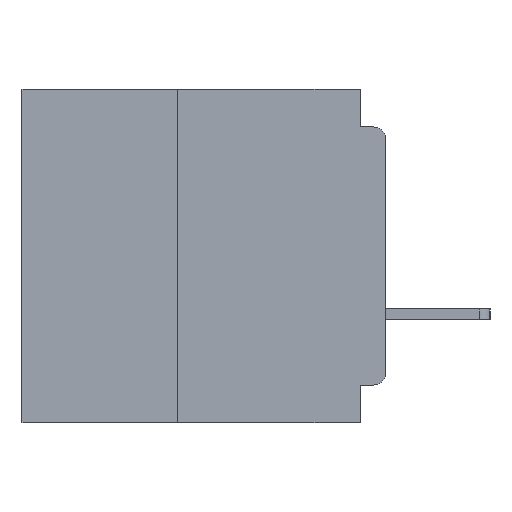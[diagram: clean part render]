
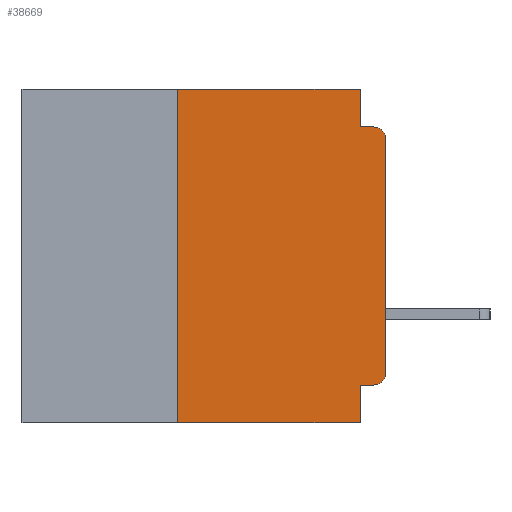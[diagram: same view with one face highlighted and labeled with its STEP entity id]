
A CAD part, left-side view. The second image highlights one B-rep face of the part: STEP entity #38669.
In plain terms, the highlighted planar face has unit normal (-1, 0, 0).
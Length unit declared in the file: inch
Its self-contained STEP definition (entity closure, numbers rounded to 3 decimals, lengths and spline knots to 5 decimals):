
#1066 = CARTESIAN_POINT ( 'NONE',  ( 0., 0., -0.34 ) ) ;
#1947 = CARTESIAN_POINT ( 'NONE',  ( 0., 0.015, -0.355 ) ) ;
#2549 = DIRECTION ( 'NONE',  ( 0., 1., 0. ) ) ;
#3871 = EDGE_CURVE ( 'NONE', #40493, #19593, #13077, .T. ) ;
#4019 = CARTESIAN_POINT ( 'NONE',  ( 0., 0.437, 0. ) ) ;
#4484 = LINE ( 'NONE', #27538, #34651 ) ;
#5518 = CARTESIAN_POINT ( 'NONE',  ( 0., 0.031, -0.045 ) ) ;
#5883 = ORIENTED_EDGE ( 'NONE', *, *, #23034, .T. ) ;
#6150 = VERTEX_POINT ( 'NONE', #48882 ) ;
#6735 = CARTESIAN_POINT ( 'NONE',  ( 0., 0.031, 0. ) ) ;
#6965 = VECTOR ( 'NONE', #24203, 39.37008 ) ;
#7120 = ORIENTED_EDGE ( 'NONE', *, *, #12433, .F. ) ;
#7440 = VERTEX_POINT ( 'NONE', #21832 ) ;
#7497 = EDGE_CURVE ( 'NONE', #41842, #40420, #8061, .T. ) ;
#8061 = CIRCLE ( 'NONE', #9426, 0.015 ) ;
#9426 = AXIS2_PLACEMENT_3D ( 'NONE', #37929, #14383, #41852 ) ;
#10115 = CARTESIAN_POINT ( 'NONE',  ( 0., 0.25, -0.4 ) ) ;
#10755 = VERTEX_POINT ( 'NONE', #10769 ) ;
#10769 = CARTESIAN_POINT ( 'NONE',  ( 0., 0.031, -0.355 ) ) ;
#10851 = ORIENTED_EDGE ( 'NONE', *, *, #26027, .F. ) ;
#11291 = VECTOR ( 'NONE', #14084, 39.37008 ) ;
#11478 = CIRCLE ( 'NONE', #41510, 0.015 ) ;
#11976 = DIRECTION ( 'NONE',  ( 0., 0., -1. ) ) ;
#12433 = EDGE_CURVE ( 'NONE', #10755, #6150, #41436, .T. ) ;
#12684 = ORIENTED_EDGE ( 'NONE', *, *, #38615, .F. ) ;
#13026 = VERTEX_POINT ( 'NONE', #34021 ) ;
#13043 = DIRECTION ( 'NONE',  ( -1., 0., 0. ) ) ;
#13077 = LINE ( 'NONE', #48177, #22372 ) ;
#13551 = VERTEX_POINT ( 'NONE', #29403 ) ;
#14084 = DIRECTION ( 'NONE',  ( 0., 0., 1. ) ) ;
#14383 = DIRECTION ( 'NONE',  ( -1., 0., 0. ) ) ;
#14529 = ORIENTED_EDGE ( 'NONE', *, *, #30905, .F. ) ;
#15608 = CARTESIAN_POINT ( 'NONE',  ( 0., 0.437, 0. ) ) ;
#16957 = ORIENTED_EDGE ( 'NONE', *, *, #3871, .F. ) ;
#17668 = EDGE_LOOP ( 'NONE', ( #48887, #32915, #16957, #14529, #12684, #44018, #5883, #7120, #10851, #46527 ) ) ;
#19593 = VERTEX_POINT ( 'NONE', #47287 ) ;
#20757 = EDGE_CURVE ( 'NONE', #13026, #19593, #11478, .T. ) ;
#21295 = VECTOR ( 'NONE', #38230, 39.37008 ) ;
#21832 = CARTESIAN_POINT ( 'NONE',  ( 0., 0.25, -0.4 ) ) ;
#22372 = VECTOR ( 'NONE', #50262, 39.37008 ) ;
#22408 = EDGE_CURVE ( 'NONE', #40420, #13026, #4484, .T. ) ;
#23034 = EDGE_CURVE ( 'NONE', #7440, #6150, #27948, .T. ) ;
#24203 = DIRECTION ( 'NONE',  ( 0., -1., 0. ) ) ;
#24249 = VECTOR ( 'NONE', #2549, 39.37008 ) ;
#25660 = EDGE_CURVE ( 'NONE', #7440, #13551, #32226, .T. ) ;
#25948 = CARTESIAN_POINT ( 'NONE',  ( 0., 0.031, 0. ) ) ;
#26027 = EDGE_CURVE ( 'NONE', #41842, #10755, #45028, .T. ) ;
#26260 = DIRECTION ( 'NONE',  ( 0., 0., -1. ) ) ;
#27538 = CARTESIAN_POINT ( 'NONE',  ( 0., 0., 0. ) ) ;
#27948 = LINE ( 'NONE', #47654, #6965 ) ;
#29403 = CARTESIAN_POINT ( 'NONE',  ( 0., 0.25, 0. ) ) ;
#30035 = CARTESIAN_POINT ( 'NONE',  ( 0., 0.031, -0.4 ) ) ;
#30905 = EDGE_CURVE ( 'NONE', #50402, #40493, #32927, .T. ) ;
#32226 = LINE ( 'NONE', #10115, #11291 ) ;
#32915 = ORIENTED_EDGE ( 'NONE', *, *, #20757, .T. ) ;
#32927 = LINE ( 'NONE', #6735, #21295 ) ;
#34021 = CARTESIAN_POINT ( 'NONE',  ( 0., 0., -0.06 ) ) ;
#34651 = VECTOR ( 'NONE', #35413, 39.37008 ) ;
#35413 = DIRECTION ( 'NONE',  ( 0., 0., 1. ) ) ;
#35522 = DIRECTION ( 'NONE',  ( 1., 0., 0. ) ) ;
#36426 = FACE_OUTER_BOUND ( 'NONE', #17668, .T. ) ;
#36597 = CARTESIAN_POINT ( 'NONE',  ( 0., 0.015, -0.06 ) ) ;
#37929 = CARTESIAN_POINT ( 'NONE',  ( 0., 0.015, -0.34 ) ) ;
#38230 = DIRECTION ( 'NONE',  ( 0., 0., -1. ) ) ;
#38615 = EDGE_CURVE ( 'NONE', #13551, #50402, #49348, .T. ) ;
#38669 = ADVANCED_FACE ( 'NONE', ( #36426 ), #47173, .F. ) ;
#40138 = VECTOR ( 'NONE', #43056, 39.37008 ) ;
#40420 = VERTEX_POINT ( 'NONE', #1066 ) ;
#40493 = VERTEX_POINT ( 'NONE', #5518 ) ;
#40549 = DIRECTION ( 'NONE',  ( 0., 0., -1. ) ) ;
#41436 = LINE ( 'NONE', #30035, #49416 ) ;
#41510 = AXIS2_PLACEMENT_3D ( 'NONE', #36597, #13043, #40549 ) ;
#41842 = VERTEX_POINT ( 'NONE', #1947 ) ;
#41852 = DIRECTION ( 'NONE',  ( 0., 0., -1. ) ) ;
#43056 = DIRECTION ( 'NONE',  ( 0., -1., 0. ) ) ;
#44018 = ORIENTED_EDGE ( 'NONE', *, *, #25660, .F. ) ;
#45028 = LINE ( 'NONE', #49680, #24249 ) ;
#46012 = AXIS2_PLACEMENT_3D ( 'NONE', #4019, #35522, #11976 ) ;
#46527 = ORIENTED_EDGE ( 'NONE', *, *, #7497, .T. ) ;
#47173 = PLANE ( 'NONE',  #46012 ) ;
#47287 = CARTESIAN_POINT ( 'NONE',  ( 0., 0.015, -0.045 ) ) ;
#47654 = CARTESIAN_POINT ( 'NONE',  ( 0., 0.437, -0.4 ) ) ;
#48177 = CARTESIAN_POINT ( 'NONE',  ( 0., 0., -0.045 ) ) ;
#48882 = CARTESIAN_POINT ( 'NONE',  ( 0., 0.031, -0.4 ) ) ;
#48887 = ORIENTED_EDGE ( 'NONE', *, *, #22408, .T. ) ;
#49348 = LINE ( 'NONE', #15608, #40138 ) ;
#49416 = VECTOR ( 'NONE', #26260, 39.37008 ) ;
#49680 = CARTESIAN_POINT ( 'NONE',  ( 0., 0., -0.355 ) ) ;
#50262 = DIRECTION ( 'NONE',  ( 0., -1., 0. ) ) ;
#50402 = VERTEX_POINT ( 'NONE', #25948 ) ;
